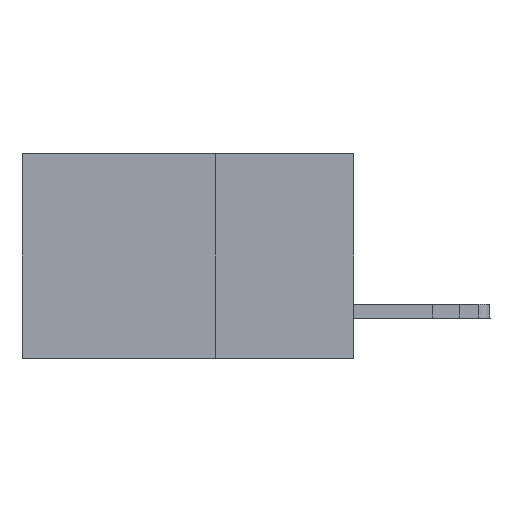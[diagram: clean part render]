
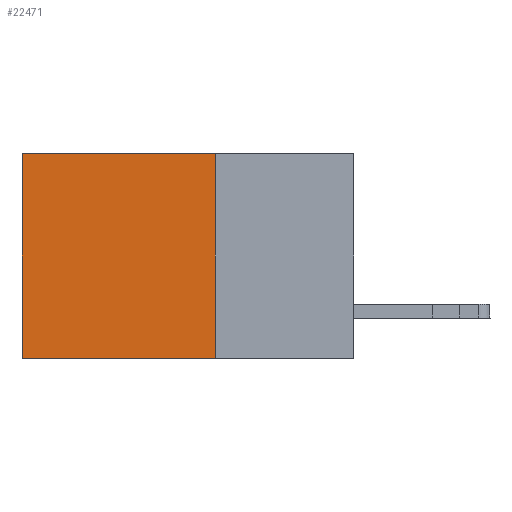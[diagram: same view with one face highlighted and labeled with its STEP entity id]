
A CAD part, left-side view. The second image highlights one B-rep face of the part: STEP entity #22471.
In plain terms, the highlighted planar face has unit normal (-1, 0, 0).
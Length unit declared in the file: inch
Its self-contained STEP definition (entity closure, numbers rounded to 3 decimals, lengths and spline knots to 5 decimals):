
#509 = LINE ( 'NONE', #24734, #20146 ) ;
#1026 = CARTESIAN_POINT ( 'NONE',  ( 0.2875, 0.6, 0. ) ) ;
#1420 = EDGE_CURVE ( 'NONE', #3373, #4184, #509, .T. ) ;
#3373 = VERTEX_POINT ( 'NONE', #1026 ) ;
#4117 = DIRECTION ( 'NONE',  ( 0., 0., -1. ) ) ;
#4184 = VERTEX_POINT ( 'NONE', #20381 ) ;
#5438 = VECTOR ( 'NONE', #25289, 39.37008 ) ;
#5793 = EDGE_CURVE ( 'NONE', #25369, #3373, #8782, .T. ) ;
#6531 = CARTESIAN_POINT ( 'NONE',  ( 0.2875, 0.25, 0. ) ) ;
#6607 = LINE ( 'NONE', #20566, #21667 ) ;
#7873 = DIRECTION ( 'NONE',  ( 0., 1., 0. ) ) ;
#8782 = LINE ( 'NONE', #13706, #22625 ) ;
#9449 = FACE_OUTER_BOUND ( 'NONE', #23193, .T. ) ;
#9574 = CARTESIAN_POINT ( 'NONE',  ( 0.2875, 0.25, -0.37 ) ) ;
#10443 = DIRECTION ( 'NONE',  ( 1., 0., 0. ) ) ;
#10590 = LINE ( 'NONE', #9574, #5438 ) ;
#10702 = DIRECTION ( 'NONE',  ( 0., 0., -1. ) ) ;
#10722 = VERTEX_POINT ( 'NONE', #14645 ) ;
#10842 = ORIENTED_EDGE ( 'NONE', *, *, #24434, .F. ) ;
#12313 = ORIENTED_EDGE ( 'NONE', *, *, #5793, .T. ) ;
#13706 = CARTESIAN_POINT ( 'NONE',  ( 0.2875, 0.25, 0. ) ) ;
#14312 = PLANE ( 'NONE',  #19890 ) ;
#14645 = CARTESIAN_POINT ( 'NONE',  ( 0.2875, 0.25, -0.37 ) ) ;
#18664 = ORIENTED_EDGE ( 'NONE', *, *, #24695, .F. ) ;
#19890 = AXIS2_PLACEMENT_3D ( 'NONE', #6531, #10443, #24211 ) ;
#20146 = VECTOR ( 'NONE', #4117, 39.37008 ) ;
#20381 = CARTESIAN_POINT ( 'NONE',  ( 0.2875, 0.6, -0.37 ) ) ;
#20566 = CARTESIAN_POINT ( 'NONE',  ( 0.2875, 0.25, 0. ) ) ;
#20880 = ORIENTED_EDGE ( 'NONE', *, *, #1420, .T. ) ;
#21667 = VECTOR ( 'NONE', #10702, 39.37008 ) ;
#21857 = CARTESIAN_POINT ( 'NONE',  ( 0.2875, 0.25, 0. ) ) ;
#22471 = ADVANCED_FACE ( 'NONE', ( #9449 ), #14312, .F. ) ;
#22625 = VECTOR ( 'NONE', #7873, 39.37008 ) ;
#23193 = EDGE_LOOP ( 'NONE', ( #20880, #18664, #10842, #12313 ) ) ;
#24211 = DIRECTION ( 'NONE',  ( 0., 0., -1. ) ) ;
#24434 = EDGE_CURVE ( 'NONE', #25369, #10722, #6607, .T. ) ;
#24695 = EDGE_CURVE ( 'NONE', #10722, #4184, #10590, .T. ) ;
#24734 = CARTESIAN_POINT ( 'NONE',  ( 0.2875, 0.6, 0. ) ) ;
#25289 = DIRECTION ( 'NONE',  ( 0., 1., 0. ) ) ;
#25369 = VERTEX_POINT ( 'NONE', #21857 ) ;
